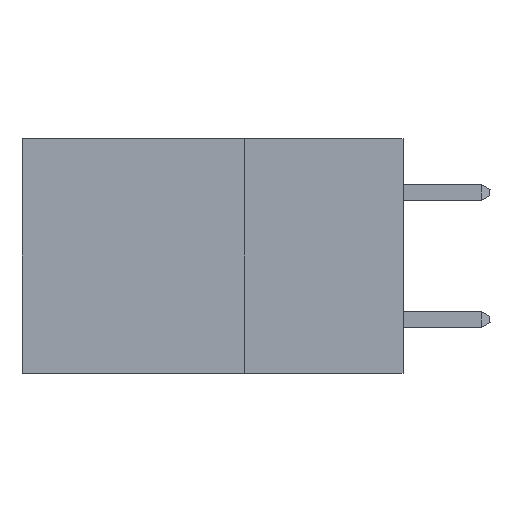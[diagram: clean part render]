
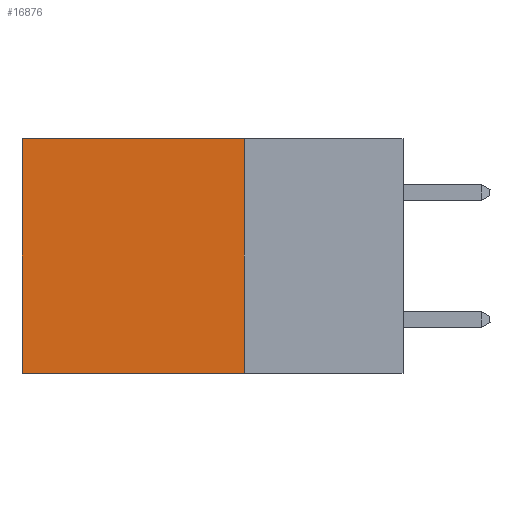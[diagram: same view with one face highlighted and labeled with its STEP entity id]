
A CAD part, left-side view. The second image highlights one B-rep face of the part: STEP entity #16876.
In plain terms, the highlighted planar face has unit normal (-1, 0, 0).
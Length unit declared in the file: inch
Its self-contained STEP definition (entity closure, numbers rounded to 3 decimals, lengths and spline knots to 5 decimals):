
#216 = ORIENTED_EDGE ( 'NONE', *, *, #9945, .F. ) ;
#1273 = ORIENTED_EDGE ( 'NONE', *, *, #6057, .F. ) ;
#1506 = LINE ( 'NONE', #5565, #11355 ) ;
#2293 = CARTESIAN_POINT ( 'NONE',  ( 0.2875, 0.25, 0. ) ) ;
#2415 = DIRECTION ( 'NONE',  ( 0., 0., -1. ) ) ;
#2456 = CARTESIAN_POINT ( 'NONE',  ( 0.2875, 0.25, -0.37 ) ) ;
#2926 = CARTESIAN_POINT ( 'NONE',  ( 0.2875, 0.6, -0.37 ) ) ;
#2935 = DIRECTION ( 'NONE',  ( 0., 1., 0. ) ) ;
#3176 = VERTEX_POINT ( 'NONE', #2926 ) ;
#4824 = LINE ( 'NONE', #2293, #15095 ) ;
#5565 = CARTESIAN_POINT ( 'NONE',  ( 0.2875, 0.6, 0. ) ) ;
#5631 = CARTESIAN_POINT ( 'NONE',  ( 0.2875, 0.6, 0. ) ) ;
#6057 = EDGE_CURVE ( 'NONE', #16879, #7671, #4824, .T. ) ;
#6627 = CARTESIAN_POINT ( 'NONE',  ( 0.2875, 0.25, 0. ) ) ;
#6690 = DIRECTION ( 'NONE',  ( 0., 1., 0. ) ) ;
#7010 = VECTOR ( 'NONE', #2935, 39.37008 ) ;
#7194 = EDGE_LOOP ( 'NONE', ( #12445, #216, #1273, #11747 ) ) ;
#7671 = VERTEX_POINT ( 'NONE', #14857 ) ;
#7922 = CARTESIAN_POINT ( 'NONE',  ( 0.2875, 0.25, 0. ) ) ;
#9113 = LINE ( 'NONE', #2456, #7010 ) ;
#9945 = EDGE_CURVE ( 'NONE', #7671, #3176, #9113, .T. ) ;
#10100 = VECTOR ( 'NONE', #6690, 39.37008 ) ;
#11355 = VECTOR ( 'NONE', #15610, 39.37008 ) ;
#11747 = ORIENTED_EDGE ( 'NONE', *, *, #11824, .T. ) ;
#11824 = EDGE_CURVE ( 'NONE', #16879, #12081, #14931, .T. ) ;
#11956 = CARTESIAN_POINT ( 'NONE',  ( 0.2875, 0.25, 0. ) ) ;
#12081 = VERTEX_POINT ( 'NONE', #5631 ) ;
#12183 = FACE_OUTER_BOUND ( 'NONE', #7194, .T. ) ;
#12445 = ORIENTED_EDGE ( 'NONE', *, *, #15195, .T. ) ;
#13354 = DIRECTION ( 'NONE',  ( 1., 0., 0. ) ) ;
#13407 = DIRECTION ( 'NONE',  ( 0., 0., -1. ) ) ;
#14857 = CARTESIAN_POINT ( 'NONE',  ( 0.2875, 0.25, -0.37 ) ) ;
#14931 = LINE ( 'NONE', #6627, #10100 ) ;
#15095 = VECTOR ( 'NONE', #2415, 39.37008 ) ;
#15195 = EDGE_CURVE ( 'NONE', #12081, #3176, #1506, .T. ) ;
#15610 = DIRECTION ( 'NONE',  ( 0., 0., -1. ) ) ;
#15933 = PLANE ( 'NONE',  #16259 ) ;
#16259 = AXIS2_PLACEMENT_3D ( 'NONE', #7922, #13354, #13407 ) ;
#16876 = ADVANCED_FACE ( 'NONE', ( #12183 ), #15933, .F. ) ;
#16879 = VERTEX_POINT ( 'NONE', #11956 ) ;
